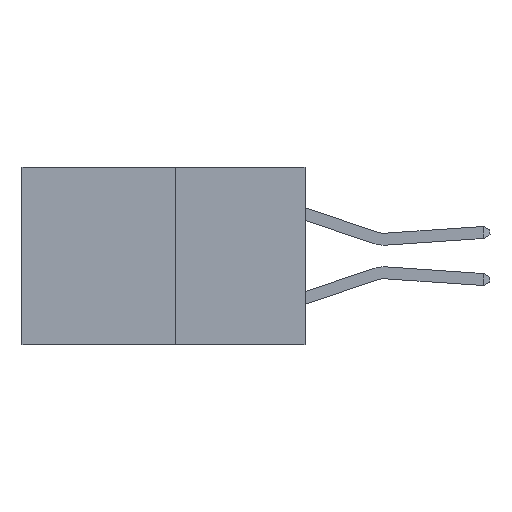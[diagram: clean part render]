
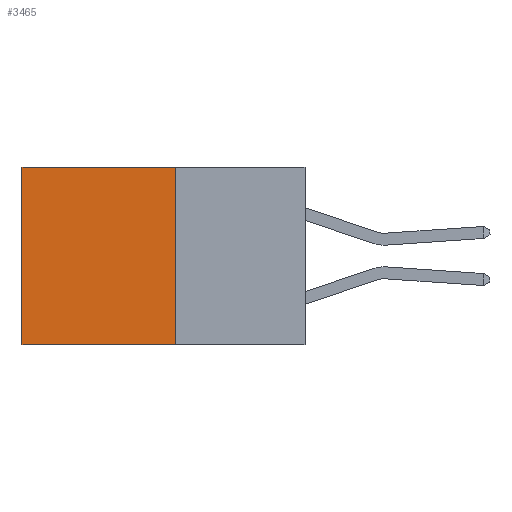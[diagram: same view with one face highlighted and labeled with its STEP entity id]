
A CAD part, left-side view. The second image highlights one B-rep face of the part: STEP entity #3465.
In plain terms, the highlighted planar face has unit normal (-1, 0, 0).
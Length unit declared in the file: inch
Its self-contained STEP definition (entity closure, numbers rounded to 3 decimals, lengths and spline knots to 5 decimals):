
#885 = VERTEX_POINT ( 'NONE', #9002 ) ;
#969 = ORIENTED_EDGE ( 'NONE', *, *, #23497, .F. ) ;
#2042 = ORIENTED_EDGE ( 'NONE', *, *, #17719, .T. ) ;
#3465 = ADVANCED_FACE ( 'NONE', ( #15035 ), #8954, .F. ) ;
#4453 = LINE ( 'NONE', #11395, #23546 ) ;
#5124 = VERTEX_POINT ( 'NONE', #15827 ) ;
#5945 = CARTESIAN_POINT ( 'NONE',  ( 0.277, 0.59, 0. ) ) ;
#6096 = LINE ( 'NONE', #18155, #11117 ) ;
#6402 = LINE ( 'NONE', #7719, #20021 ) ;
#7320 = EDGE_LOOP ( 'NONE', ( #14552, #969, #19100, #2042 ) ) ;
#7606 = CARTESIAN_POINT ( 'NONE',  ( 0.277, 0.27, 0. ) ) ;
#7719 = CARTESIAN_POINT ( 'NONE',  ( 0.277, 0.27, -0.37 ) ) ;
#8949 = DIRECTION ( 'NONE',  ( 0., 0., -1. ) ) ;
#8954 = PLANE ( 'NONE',  #13851 ) ;
#9002 = CARTESIAN_POINT ( 'NONE',  ( 0.277, 0.27, 0. ) ) ;
#10746 = DIRECTION ( 'NONE',  ( 1., 0., 0. ) ) ;
#11117 = VECTOR ( 'NONE', #8949, 39.37008 ) ;
#11186 = CARTESIAN_POINT ( 'NONE',  ( 0.277, 0.27, -0.37 ) ) ;
#11395 = CARTESIAN_POINT ( 'NONE',  ( 0.277, 0.27, -0.37 ) ) ;
#11767 = DIRECTION ( 'NONE',  ( 0., 0., -1. ) ) ;
#12371 = EDGE_CURVE ( 'NONE', #23545, #18815, #6096, .T. ) ;
#12493 = CARTESIAN_POINT ( 'NONE',  ( 0.277, 0.59, -0.37 ) ) ;
#13851 = AXIS2_PLACEMENT_3D ( 'NONE', #11186, #10746, #11767 ) ;
#14304 = VECTOR ( 'NONE', #20535, 39.37008 ) ;
#14552 = ORIENTED_EDGE ( 'NONE', *, *, #12371, .T. ) ;
#14901 = LINE ( 'NONE', #7606, #14304 ) ;
#15035 = FACE_OUTER_BOUND ( 'NONE', #7320, .T. ) ;
#15827 = CARTESIAN_POINT ( 'NONE',  ( 0.277, 0.27, -0.37 ) ) ;
#17062 = EDGE_CURVE ( 'NONE', #885, #5124, #6402, .T. ) ;
#17719 = EDGE_CURVE ( 'NONE', #885, #23545, #14901, .T. ) ;
#18155 = CARTESIAN_POINT ( 'NONE',  ( 0.277, 0.59, -0.37 ) ) ;
#18804 = DIRECTION ( 'NONE',  ( 0., 0., -1. ) ) ;
#18815 = VERTEX_POINT ( 'NONE', #12493 ) ;
#19100 = ORIENTED_EDGE ( 'NONE', *, *, #17062, .F. ) ;
#20021 = VECTOR ( 'NONE', #18804, 39.37008 ) ;
#20535 = DIRECTION ( 'NONE',  ( 0., 1., 0. ) ) ;
#22359 = DIRECTION ( 'NONE',  ( 0., 1., 0. ) ) ;
#23497 = EDGE_CURVE ( 'NONE', #5124, #18815, #4453, .T. ) ;
#23545 = VERTEX_POINT ( 'NONE', #5945 ) ;
#23546 = VECTOR ( 'NONE', #22359, 39.37008 ) ;
